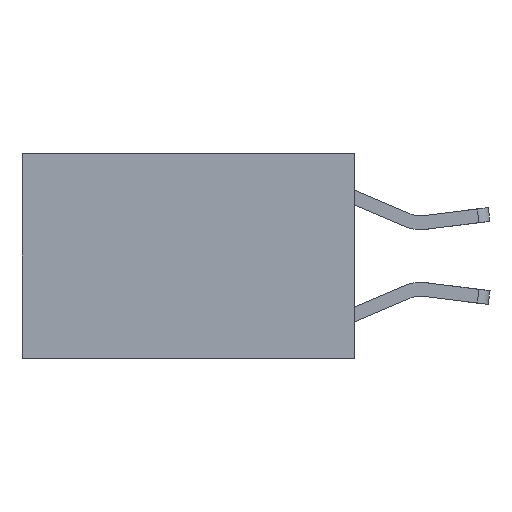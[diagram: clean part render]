
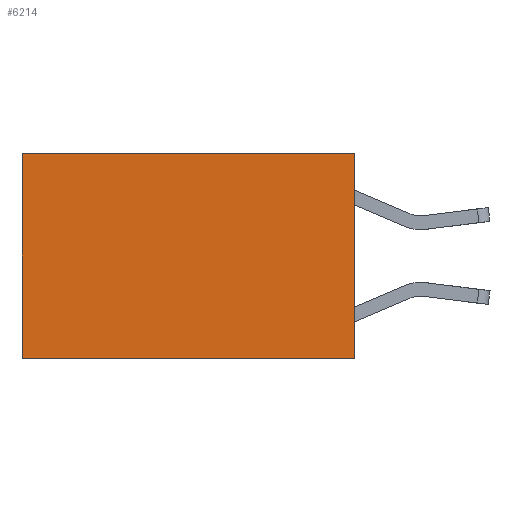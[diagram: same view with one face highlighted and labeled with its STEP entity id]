
A CAD part, left-side view. The second image highlights one B-rep face of the part: STEP entity #6214.
In plain terms, the highlighted planar face has unit normal (-1, 0, 0).
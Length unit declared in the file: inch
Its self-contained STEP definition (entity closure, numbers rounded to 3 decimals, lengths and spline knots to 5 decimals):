
#178 = CARTESIAN_POINT ( 'NONE',  ( 0.2625, 0., 0. ) ) ;
#859 = FACE_OUTER_BOUND ( 'NONE', #1727, .T. ) ;
#1199 = CARTESIAN_POINT ( 'NONE',  ( 0.2625, 0., 0. ) ) ;
#1659 = LINE ( 'NONE', #9612, #7921 ) ;
#1727 = EDGE_LOOP ( 'NONE', ( #7312, #5958, #9824, #6527 ) ) ;
#1931 = CARTESIAN_POINT ( 'NONE',  ( 0.2625, 0.6, 0. ) ) ;
#2217 = VERTEX_POINT ( 'NONE', #178 ) ;
#2750 = LINE ( 'NONE', #1199, #7609 ) ;
#2841 = VERTEX_POINT ( 'NONE', #7910 ) ;
#3668 = CARTESIAN_POINT ( 'NONE',  ( 0.2625, 0., 0. ) ) ;
#4855 = EDGE_CURVE ( 'NONE', #2217, #8959, #2750, .T. ) ;
#5074 = VECTOR ( 'NONE', #8592, 39.37008 ) ;
#5958 = ORIENTED_EDGE ( 'NONE', *, *, #7452, .F. ) ;
#5986 = DIRECTION ( 'NONE',  ( 0., 1., 0. ) ) ;
#6036 = PLANE ( 'NONE',  #8783 ) ;
#6214 = ADVANCED_FACE ( 'NONE', ( #859 ), #6036, .F. ) ;
#6281 = CARTESIAN_POINT ( 'NONE',  ( 0.2625, 0.6, -0.37 ) ) ;
#6527 = ORIENTED_EDGE ( 'NONE', *, *, #4855, .T. ) ;
#6792 = DIRECTION ( 'NONE',  ( 1., 0., 0. ) ) ;
#7279 = VECTOR ( 'NONE', #7846, 39.37008 ) ;
#7312 = ORIENTED_EDGE ( 'NONE', *, *, #9367, .T. ) ;
#7452 = EDGE_CURVE ( 'NONE', #2841, #8226, #8703, .T. ) ;
#7609 = VECTOR ( 'NONE', #5986, 39.37008 ) ;
#7835 = DIRECTION ( 'NONE',  ( 0., 0., -1. ) ) ;
#7846 = DIRECTION ( 'NONE',  ( 0., 0., -1. ) ) ;
#7910 = CARTESIAN_POINT ( 'NONE',  ( 0.2625, 0., -0.37 ) ) ;
#7921 = VECTOR ( 'NONE', #7835, 39.37008 ) ;
#8226 = VERTEX_POINT ( 'NONE', #6281 ) ;
#8457 = DIRECTION ( 'NONE',  ( 0., 0., -1. ) ) ;
#8592 = DIRECTION ( 'NONE',  ( 0., 1., 0. ) ) ;
#8666 = CARTESIAN_POINT ( 'NONE',  ( 0.2625, 0., -0.37 ) ) ;
#8703 = LINE ( 'NONE', #8666, #5074 ) ;
#8783 = AXIS2_PLACEMENT_3D ( 'NONE', #3668, #6792, #8457 ) ;
#8959 = VERTEX_POINT ( 'NONE', #1931 ) ;
#9176 = EDGE_CURVE ( 'NONE', #2217, #2841, #1659, .T. ) ;
#9220 = CARTESIAN_POINT ( 'NONE',  ( 0.2625, 0.6, 0. ) ) ;
#9367 = EDGE_CURVE ( 'NONE', #8959, #8226, #9452, .T. ) ;
#9452 = LINE ( 'NONE', #9220, #7279 ) ;
#9612 = CARTESIAN_POINT ( 'NONE',  ( 0.2625, 0., 0. ) ) ;
#9824 = ORIENTED_EDGE ( 'NONE', *, *, #9176, .F. ) ;
